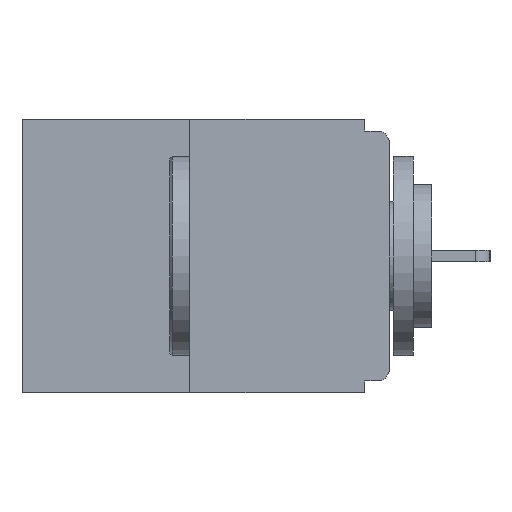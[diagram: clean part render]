
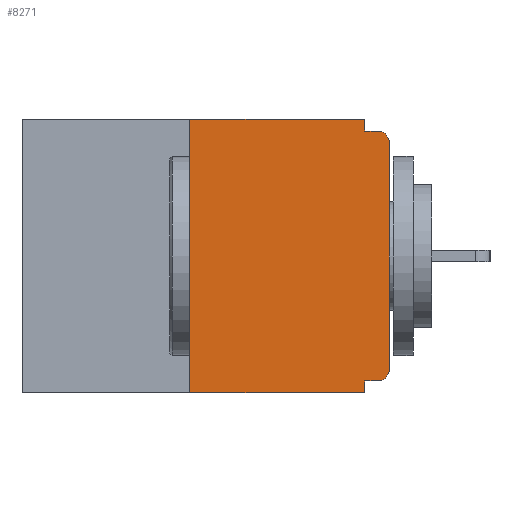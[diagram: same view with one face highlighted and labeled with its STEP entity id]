
A CAD part, left-side view. The second image highlights one B-rep face of the part: STEP entity #8271.
In plain terms, the highlighted planar face has unit normal (-1, 0, 0).
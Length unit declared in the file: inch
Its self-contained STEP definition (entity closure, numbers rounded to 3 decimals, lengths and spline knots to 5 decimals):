
#168 = VERTEX_POINT ( 'NONE', #1302 ) ;
#186 = VERTEX_POINT ( 'NONE', #13808 ) ;
#205 = LINE ( 'NONE', #6701, #9855 ) ;
#238 = VECTOR ( 'NONE', #5597, 39.37008 ) ;
#374 = VECTOR ( 'NONE', #777, 39.37008 ) ;
#517 = CARTESIAN_POINT ( 'NONE',  ( 0., 0., -0.328 ) ) ;
#554 = EDGE_CURVE ( 'NONE', #12922, #13567, #205, .T. ) ;
#755 = VERTEX_POINT ( 'NONE', #4564 ) ;
#777 = DIRECTION ( 'NONE',  ( 0., -1., 0. ) ) ;
#1139 = EDGE_CURVE ( 'NONE', #755, #14903, #8690, .T. ) ;
#1185 = VERTEX_POINT ( 'NONE', #12679 ) ;
#1302 = CARTESIAN_POINT ( 'NONE',  ( 0., 0., -0.03 ) ) ;
#1437 = LINE ( 'NONE', #6065, #7522 ) ;
#1531 = DIRECTION ( 'NONE',  ( 0., -1., 0. ) ) ;
#1951 = EDGE_CURVE ( 'NONE', #13567, #186, #13652, .T. ) ;
#2015 = CARTESIAN_POINT ( 'NONE',  ( 0., 0.46, 0. ) ) ;
#2030 = VECTOR ( 'NONE', #7734, 39.37008 ) ;
#2279 = CARTESIAN_POINT ( 'NONE',  ( 0., 0.031, 0. ) ) ;
#2739 = EDGE_CURVE ( 'NONE', #8196, #755, #15121, .T. ) ;
#3085 = ORIENTED_EDGE ( 'NONE', *, *, #554, .F. ) ;
#3202 = EDGE_CURVE ( 'NONE', #186, #1185, #5477, .T. ) ;
#3672 = CARTESIAN_POINT ( 'NONE',  ( 0., 0.015, -0.313 ) ) ;
#3767 = VERTEX_POINT ( 'NONE', #4843 ) ;
#3907 = ORIENTED_EDGE ( 'NONE', *, *, #7565, .T. ) ;
#4309 = ORIENTED_EDGE ( 'NONE', *, *, #10752, .T. ) ;
#4564 = CARTESIAN_POINT ( 'NONE',  ( 0., 0.031, -0.328 ) ) ;
#4798 = PLANE ( 'NONE',  #11275 ) ;
#4843 = CARTESIAN_POINT ( 'NONE',  ( 0., 0.015, -0.015 ) ) ;
#4974 = DIRECTION ( 'NONE',  ( 0., 0., -1. ) ) ;
#5066 = CARTESIAN_POINT ( 'NONE',  ( 0., 0.031, -0.343 ) ) ;
#5324 = VECTOR ( 'NONE', #15278, 39.37008 ) ;
#5477 = LINE ( 'NONE', #2279, #15135 ) ;
#5597 = DIRECTION ( 'NONE',  ( 0., 0., 1. ) ) ;
#5635 = CIRCLE ( 'NONE', #6622, 0.015 ) ;
#5785 = CARTESIAN_POINT ( 'NONE',  ( 0., 0., 0. ) ) ;
#6065 = CARTESIAN_POINT ( 'NONE',  ( 0., 0.46, -0.343 ) ) ;
#6369 = VERTEX_POINT ( 'NONE', #13752 ) ;
#6558 = ORIENTED_EDGE ( 'NONE', *, *, #9470, .T. ) ;
#6622 = AXIS2_PLACEMENT_3D ( 'NONE', #7661, #15970, #8858 ) ;
#6701 = CARTESIAN_POINT ( 'NONE',  ( 0., 0.25, 0. ) ) ;
#7408 = CARTESIAN_POINT ( 'NONE',  ( 0., 0.46, 0. ) ) ;
#7522 = VECTOR ( 'NONE', #14455, 39.37008 ) ;
#7565 = EDGE_CURVE ( 'NONE', #6369, #168, #13525, .T. ) ;
#7661 = CARTESIAN_POINT ( 'NONE',  ( 0., 0.015, -0.03 ) ) ;
#7734 = DIRECTION ( 'NONE',  ( 0., 1., 0. ) ) ;
#7755 = DIRECTION ( 'NONE',  ( 0., 0., -1. ) ) ;
#7943 = EDGE_LOOP ( 'NONE', ( #9445, #3085, #6558, #9844, #8884, #13318, #3907, #4309, #10968, #8142 ) ) ;
#7975 = CARTESIAN_POINT ( 'NONE',  ( 0., 0., -0.015 ) ) ;
#8140 = CIRCLE ( 'NONE', #15607, 0.015 ) ;
#8142 = ORIENTED_EDGE ( 'NONE', *, *, #3202, .F. ) ;
#8196 = VERTEX_POINT ( 'NONE', #15526 ) ;
#8271 = ADVANCED_FACE ( 'NONE', ( #12605 ), #4798, .F. ) ;
#8386 = VECTOR ( 'NONE', #1531, 39.37008 ) ;
#8614 = CARTESIAN_POINT ( 'NONE',  ( 0., 0.25, 0. ) ) ;
#8633 = DIRECTION ( 'NONE',  ( 0., 0., -1. ) ) ;
#8690 = LINE ( 'NONE', #14702, #5324 ) ;
#8858 = DIRECTION ( 'NONE',  ( 0., 0., -1. ) ) ;
#8884 = ORIENTED_EDGE ( 'NONE', *, *, #2739, .F. ) ;
#8906 = DIRECTION ( 'NONE',  ( 0., 0., 1. ) ) ;
#9445 = ORIENTED_EDGE ( 'NONE', *, *, #1951, .F. ) ;
#9470 = EDGE_CURVE ( 'NONE', #12922, #14903, #1437, .T. ) ;
#9844 = ORIENTED_EDGE ( 'NONE', *, *, #1139, .F. ) ;
#9855 = VECTOR ( 'NONE', #8906, 39.37008 ) ;
#10752 = EDGE_CURVE ( 'NONE', #168, #3767, #5635, .T. ) ;
#10968 = ORIENTED_EDGE ( 'NONE', *, *, #15793, .F. ) ;
#11006 = CARTESIAN_POINT ( 'NONE',  ( 0., 0.25, -0.343 ) ) ;
#11275 = AXIS2_PLACEMENT_3D ( 'NONE', #7408, #15739, #8633 ) ;
#11923 = LINE ( 'NONE', #7975, #8386 ) ;
#12324 = DIRECTION ( 'NONE',  ( -1., 0., 0. ) ) ;
#12605 = FACE_OUTER_BOUND ( 'NONE', #7943, .T. ) ;
#12679 = CARTESIAN_POINT ( 'NONE',  ( 0., 0.031, -0.015 ) ) ;
#12922 = VERTEX_POINT ( 'NONE', #11006 ) ;
#13318 = ORIENTED_EDGE ( 'NONE', *, *, #14226, .T. ) ;
#13525 = LINE ( 'NONE', #5785, #238 ) ;
#13567 = VERTEX_POINT ( 'NONE', #8614 ) ;
#13652 = LINE ( 'NONE', #2015, #374 ) ;
#13752 = CARTESIAN_POINT ( 'NONE',  ( 0., 0., -0.313 ) ) ;
#13808 = CARTESIAN_POINT ( 'NONE',  ( 0., 0.031, 0. ) ) ;
#14226 = EDGE_CURVE ( 'NONE', #8196, #6369, #8140, .T. ) ;
#14455 = DIRECTION ( 'NONE',  ( 0., -1., 0. ) ) ;
#14702 = CARTESIAN_POINT ( 'NONE',  ( 0., 0.031, -0.343 ) ) ;
#14903 = VERTEX_POINT ( 'NONE', #5066 ) ;
#15121 = LINE ( 'NONE', #517, #2030 ) ;
#15135 = VECTOR ( 'NONE', #7755, 39.37008 ) ;
#15278 = DIRECTION ( 'NONE',  ( 0., 0., -1. ) ) ;
#15526 = CARTESIAN_POINT ( 'NONE',  ( 0., 0.015, -0.328 ) ) ;
#15607 = AXIS2_PLACEMENT_3D ( 'NONE', #3672, #12324, #4974 ) ;
#15739 = DIRECTION ( 'NONE',  ( 1., 0., 0. ) ) ;
#15793 = EDGE_CURVE ( 'NONE', #1185, #3767, #11923, .T. ) ;
#15970 = DIRECTION ( 'NONE',  ( -1., 0., 0. ) ) ;
